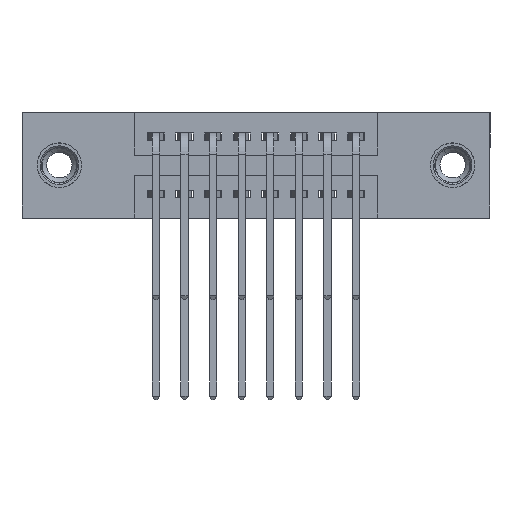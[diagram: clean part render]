
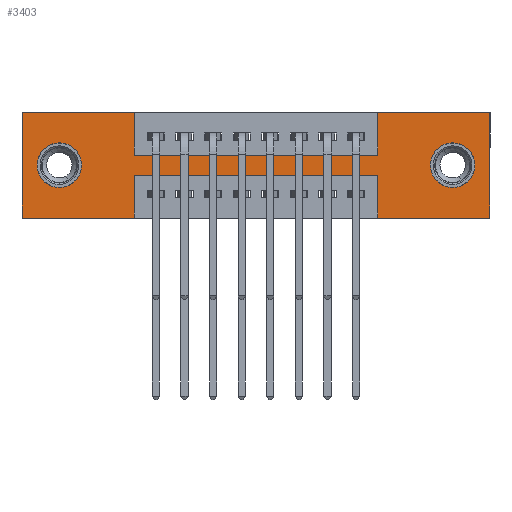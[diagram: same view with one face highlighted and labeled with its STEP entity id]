
A CAD part, front view. The second image highlights one B-rep face of the part: STEP entity #3403.
In plain terms, the highlighted planar face has unit normal (0, -1, 0).
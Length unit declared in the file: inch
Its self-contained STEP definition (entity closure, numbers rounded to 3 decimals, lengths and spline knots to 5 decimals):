
#479 = DIRECTION ( 'NONE',  ( -1., 0., 0. ) ) ;
#827 = CARTESIAN_POINT ( 'NONE',  ( 0., 0., -0.37 ) ) ;
#996 = CIRCLE ( 'NONE', #6534, 0.078 ) ;
#1112 = CARTESIAN_POINT ( 'NONE',  ( 0., 0., 0. ) ) ;
#1121 = EDGE_LOOP ( 'NONE', ( #14605, #8064 ) ) ;
#1150 = VECTOR ( 'NONE', #10457, 39.37008 ) ;
#1488 = ORIENTED_EDGE ( 'NONE', *, *, #7408, .F. ) ;
#1521 = AXIS2_PLACEMENT_3D ( 'NONE', #2132, #11487, #6156 ) ;
#1903 = CARTESIAN_POINT ( 'NONE',  ( 0.13, 0., -0.107 ) ) ;
#1927 = EDGE_CURVE ( 'NONE', #8850, #9904, #6317, .T. ) ;
#1965 = ORIENTED_EDGE ( 'NONE', *, *, #7287, .F. ) ;
#2122 = DIRECTION ( 'NONE',  ( 0., 0., 1. ) ) ;
#2132 = CARTESIAN_POINT ( 'NONE',  ( 1.505, 0., -0.185 ) ) ;
#2717 = ORIENTED_EDGE ( 'NONE', *, *, #7232, .F. ) ;
#2737 = CARTESIAN_POINT ( 'NONE',  ( 1.2425, 0., 0. ) ) ;
#2754 = FACE_BOUND ( 'NONE', #1121, .T. ) ;
#2772 = ORIENTED_EDGE ( 'NONE', *, *, #11820, .F. ) ;
#2845 = LINE ( 'NONE', #11913, #13934 ) ;
#3403 = ADVANCED_FACE ( 'NONE', ( #2754, #13002, #4615 ), #14128, .T. ) ;
#3783 = VERTEX_POINT ( 'NONE', #10250 ) ;
#3794 = EDGE_CURVE ( 'NONE', #14795, #5164, #7097, .T. ) ;
#3866 = LINE ( 'NONE', #4834, #14104 ) ;
#3872 = VERTEX_POINT ( 'NONE', #6643 ) ;
#3888 = LINE ( 'NONE', #8756, #4913 ) ;
#4051 = EDGE_CURVE ( 'NONE', #5804, #16061, #8998, .T. ) ;
#4356 = VECTOR ( 'NONE', #12777, 39.37008 ) ;
#4385 = VERTEX_POINT ( 'NONE', #7423 ) ;
#4570 = EDGE_CURVE ( 'NONE', #6164, #10969, #8770, .T. ) ;
#4615 = FACE_OUTER_BOUND ( 'NONE', #15275, .T. ) ;
#4681 = LINE ( 'NONE', #1112, #1150 ) ;
#4834 = CARTESIAN_POINT ( 'NONE',  ( 1.2425, 0., -0.37 ) ) ;
#4852 = VECTOR ( 'NONE', #14477, 39.37008 ) ;
#4913 = VECTOR ( 'NONE', #8695, 39.37008 ) ;
#5010 = ORIENTED_EDGE ( 'NONE', *, *, #9649, .F. ) ;
#5039 = DIRECTION ( 'NONE',  ( 0., 0., -1. ) ) ;
#5040 = LINE ( 'NONE', #9107, #4852 ) ;
#5164 = VERTEX_POINT ( 'NONE', #13470 ) ;
#5207 = CARTESIAN_POINT ( 'NONE',  ( 0., 0., 0. ) ) ;
#5311 = LINE ( 'NONE', #7348, #12248 ) ;
#5546 = CARTESIAN_POINT ( 'NONE',  ( 0.3925, 0., -0.15 ) ) ;
#5590 = CARTESIAN_POINT ( 'NONE',  ( 0.3925, 0., -0.37 ) ) ;
#5598 = VECTOR ( 'NONE', #8062, 39.37008 ) ;
#5804 = VERTEX_POINT ( 'NONE', #5207 ) ;
#5919 = CARTESIAN_POINT ( 'NONE',  ( 1.505, 0., -0.263 ) ) ;
#6037 = AXIS2_PLACEMENT_3D ( 'NONE', #6152, #12892, #2122 ) ;
#6152 = CARTESIAN_POINT ( 'NONE',  ( 0.13, 0., -0.185 ) ) ;
#6156 = DIRECTION ( 'NONE',  ( 0., 0., -1. ) ) ;
#6164 = VERTEX_POINT ( 'NONE', #14816 ) ;
#6317 = LINE ( 'NONE', #11107, #8636 ) ;
#6339 = ORIENTED_EDGE ( 'NONE', *, *, #4051, .F. ) ;
#6534 = AXIS2_PLACEMENT_3D ( 'NONE', #16991, #11730, #5039 ) ;
#6643 = CARTESIAN_POINT ( 'NONE',  ( 0., 0., -0.37 ) ) ;
#6852 = CARTESIAN_POINT ( 'NONE',  ( 1.635, 0., -0.37 ) ) ;
#6947 = CARTESIAN_POINT ( 'NONE',  ( 0.3925, 0., 0. ) ) ;
#7052 = CARTESIAN_POINT ( 'NONE',  ( 0.13, 0., -0.185 ) ) ;
#7097 = CIRCLE ( 'NONE', #1521, 0.078 ) ;
#7232 = EDGE_CURVE ( 'NONE', #17176, #14587, #5311, .T. ) ;
#7287 = EDGE_CURVE ( 'NONE', #14587, #8850, #3866, .T. ) ;
#7348 = CARTESIAN_POINT ( 'NONE',  ( 0., 0., -0.37 ) ) ;
#7408 = EDGE_CURVE ( 'NONE', #10969, #14483, #4681, .T. ) ;
#7423 = CARTESIAN_POINT ( 'NONE',  ( 0.13, 0., -0.263 ) ) ;
#7510 = VECTOR ( 'NONE', #13799, 39.37008 ) ;
#7610 = CARTESIAN_POINT ( 'NONE',  ( 1.2425, 0., -0.22 ) ) ;
#7742 = EDGE_CURVE ( 'NONE', #16061, #13376, #14331, .T. ) ;
#8062 = DIRECTION ( 'NONE',  ( 0., 0., -1. ) ) ;
#8064 = ORIENTED_EDGE ( 'NONE', *, *, #3794, .T. ) ;
#8143 = VERTEX_POINT ( 'NONE', #1903 ) ;
#8145 = LINE ( 'NONE', #8860, #4356 ) ;
#8333 = CIRCLE ( 'NONE', #16719, 0.078 ) ;
#8413 = CARTESIAN_POINT ( 'NONE',  ( 0., 0., 0. ) ) ;
#8500 = ORIENTED_EDGE ( 'NONE', *, *, #15679, .F. ) ;
#8636 = VECTOR ( 'NONE', #479, 39.37008 ) ;
#8695 = DIRECTION ( 'NONE',  ( 1., 0., 0. ) ) ;
#8756 = CARTESIAN_POINT ( 'NONE',  ( 0.3925, 0., -0.15 ) ) ;
#8770 = LINE ( 'NONE', #2737, #10011 ) ;
#8850 = VERTEX_POINT ( 'NONE', #7610 ) ;
#8860 = CARTESIAN_POINT ( 'NONE',  ( 0., 0., 0. ) ) ;
#8871 = EDGE_CURVE ( 'NONE', #5164, #14795, #996, .T. ) ;
#8998 = LINE ( 'NONE', #8413, #7510 ) ;
#9050 = EDGE_CURVE ( 'NONE', #3783, #3872, #2845, .T. ) ;
#9107 = CARTESIAN_POINT ( 'NONE',  ( 1.635, 0., 0. ) ) ;
#9280 = DIRECTION ( 'NONE',  ( 0., 0., -1. ) ) ;
#9649 = EDGE_CURVE ( 'NONE', #13376, #6164, #3888, .T. ) ;
#9904 = VERTEX_POINT ( 'NONE', #13632 ) ;
#10011 = VECTOR ( 'NONE', #17185, 39.37008 ) ;
#10250 = CARTESIAN_POINT ( 'NONE',  ( 0.3925, 0., -0.37 ) ) ;
#10385 = CARTESIAN_POINT ( 'NONE',  ( 1.635, 0., 0. ) ) ;
#10444 = ORIENTED_EDGE ( 'NONE', *, *, #12614, .T. ) ;
#10457 = DIRECTION ( 'NONE',  ( 1., 0., 0. ) ) ;
#10621 = DIRECTION ( 'NONE',  ( -1., 0., 0. ) ) ;
#10803 = CARTESIAN_POINT ( 'NONE',  ( 1.2425, 0., 0. ) ) ;
#10969 = VERTEX_POINT ( 'NONE', #10803 ) ;
#11107 = CARTESIAN_POINT ( 'NONE',  ( 0.3925, 0., -0.22 ) ) ;
#11160 = ORIENTED_EDGE ( 'NONE', *, *, #4570, .F. ) ;
#11387 = EDGE_LOOP ( 'NONE', ( #10444, #14887 ) ) ;
#11487 = DIRECTION ( 'NONE',  ( 0., 1., 0. ) ) ;
#11730 = DIRECTION ( 'NONE',  ( 0., 1., 0. ) ) ;
#11820 = EDGE_CURVE ( 'NONE', #14483, #17176, #5040, .T. ) ;
#11913 = CARTESIAN_POINT ( 'NONE',  ( 0., 0., -0.37 ) ) ;
#12248 = VECTOR ( 'NONE', #12747, 39.37008 ) ;
#12419 = CARTESIAN_POINT ( 'NONE',  ( 0.3925, 0., 0. ) ) ;
#12461 = VECTOR ( 'NONE', #15920, 39.37008 ) ;
#12614 = EDGE_CURVE ( 'NONE', #8143, #4385, #17170, .T. ) ;
#12747 = DIRECTION ( 'NONE',  ( -1., 0., 0. ) ) ;
#12777 = DIRECTION ( 'NONE',  ( 0., 0., 1. ) ) ;
#12892 = DIRECTION ( 'NONE',  ( 0., 1., 0. ) ) ;
#13002 = FACE_BOUND ( 'NONE', #11387, .T. ) ;
#13229 = ORIENTED_EDGE ( 'NONE', *, *, #7742, .F. ) ;
#13254 = EDGE_CURVE ( 'NONE', #3872, #5804, #8145, .T. ) ;
#13376 = VERTEX_POINT ( 'NONE', #5546 ) ;
#13420 = CARTESIAN_POINT ( 'NONE',  ( 1.2425, 0., -0.37 ) ) ;
#13470 = CARTESIAN_POINT ( 'NONE',  ( 1.505, 0., -0.107 ) ) ;
#13477 = DIRECTION ( 'NONE',  ( 0., -1., 0. ) ) ;
#13566 = LINE ( 'NONE', #5590, #5598 ) ;
#13632 = CARTESIAN_POINT ( 'NONE',  ( 0.3925, 0., -0.22 ) ) ;
#13799 = DIRECTION ( 'NONE',  ( 1., 0., 0. ) ) ;
#13934 = VECTOR ( 'NONE', #10621, 39.37008 ) ;
#14104 = VECTOR ( 'NONE', #15524, 39.37008 ) ;
#14128 = PLANE ( 'NONE',  #15062 ) ;
#14331 = LINE ( 'NONE', #6947, #12461 ) ;
#14477 = DIRECTION ( 'NONE',  ( 0., 0., -1. ) ) ;
#14483 = VERTEX_POINT ( 'NONE', #10385 ) ;
#14587 = VERTEX_POINT ( 'NONE', #13420 ) ;
#14605 = ORIENTED_EDGE ( 'NONE', *, *, #8871, .T. ) ;
#14795 = VERTEX_POINT ( 'NONE', #5919 ) ;
#14816 = CARTESIAN_POINT ( 'NONE',  ( 1.2425, 0., -0.15 ) ) ;
#14887 = ORIENTED_EDGE ( 'NONE', *, *, #15810, .T. ) ;
#15062 = AXIS2_PLACEMENT_3D ( 'NONE', #827, #13477, #9280 ) ;
#15170 = DIRECTION ( 'NONE',  ( 0., 1., 0. ) ) ;
#15275 = EDGE_LOOP ( 'NONE', ( #8500, #16359, #1965, #2717, #2772, #1488, #11160, #5010, #13229, #6339, #15302, #16027 ) ) ;
#15302 = ORIENTED_EDGE ( 'NONE', *, *, #13254, .F. ) ;
#15524 = DIRECTION ( 'NONE',  ( 0., 0., 1. ) ) ;
#15679 = EDGE_CURVE ( 'NONE', #9904, #3783, #13566, .T. ) ;
#15810 = EDGE_CURVE ( 'NONE', #4385, #8143, #8333, .T. ) ;
#15920 = DIRECTION ( 'NONE',  ( 0., 0., -1. ) ) ;
#16027 = ORIENTED_EDGE ( 'NONE', *, *, #9050, .F. ) ;
#16061 = VERTEX_POINT ( 'NONE', #12419 ) ;
#16359 = ORIENTED_EDGE ( 'NONE', *, *, #1927, .F. ) ;
#16419 = DIRECTION ( 'NONE',  ( 0., 0., 1. ) ) ;
#16719 = AXIS2_PLACEMENT_3D ( 'NONE', #7052, #15170, #16419 ) ;
#16991 = CARTESIAN_POINT ( 'NONE',  ( 1.505, 0., -0.185 ) ) ;
#17170 = CIRCLE ( 'NONE', #6037, 0.078 ) ;
#17176 = VERTEX_POINT ( 'NONE', #6852 ) ;
#17185 = DIRECTION ( 'NONE',  ( 0., 0., 1. ) ) ;
